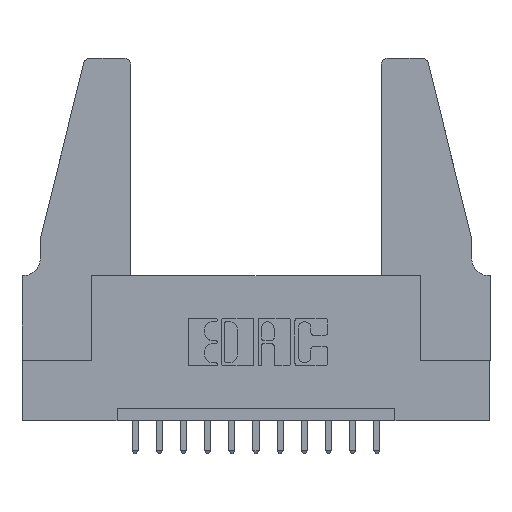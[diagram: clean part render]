
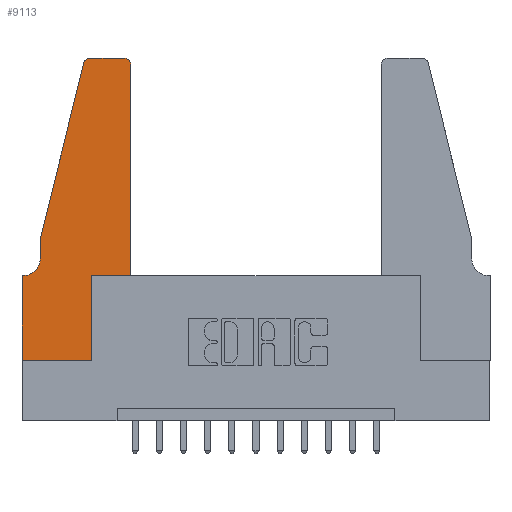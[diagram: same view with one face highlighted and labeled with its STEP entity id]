
A CAD part, top view. The second image highlights one B-rep face of the part: STEP entity #9113.
In plain terms, the highlighted planar face has unit normal (0, 0, 1).
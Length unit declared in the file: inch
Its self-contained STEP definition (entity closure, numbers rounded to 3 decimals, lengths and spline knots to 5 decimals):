
#125 = CARTESIAN_POINT ( 'NONE',  ( 0., 0., 0.37 ) ) ;
#191 = CARTESIAN_POINT ( 'NONE',  ( 0.2865, 0.35, 0.37 ) ) ;
#464 = EDGE_CURVE ( 'NONE', #8051, #4748, #11514, .T. ) ;
#526 = DIRECTION ( 'NONE',  ( 1., 0., 0. ) ) ;
#865 = CARTESIAN_POINT ( 'NONE',  ( 0.2605, 1.25, 0.37 ) ) ;
#1005 = CARTESIAN_POINT ( 'NONE',  ( 0.0755, 0.5, 0.37 ) ) ;
#1082 = AXIS2_PLACEMENT_3D ( 'NONE', #11860, #1566, #526 ) ;
#1183 = VERTEX_POINT ( 'NONE', #7033 ) ;
#1487 = LINE ( 'NONE', #8215, #7141 ) ;
#1566 = DIRECTION ( 'NONE',  ( 0., 0., 1. ) ) ;
#1735 = ORIENTED_EDGE ( 'NONE', *, *, #11050, .T. ) ;
#1861 = DIRECTION ( 'NONE',  ( -1., 0., 0. ) ) ;
#1981 = EDGE_CURVE ( 'NONE', #13325, #2441, #13966, .T. ) ;
#2212 = EDGE_CURVE ( 'NONE', #7018, #9167, #8469, .T. ) ;
#2230 = EDGE_CURVE ( 'NONE', #11353, #11783, #5502, .T. ) ;
#2374 = DIRECTION ( 'NONE',  ( 0., -1., 0. ) ) ;
#2427 = CARTESIAN_POINT ( 'NONE',  ( 0.2865, 0.35, 0.37 ) ) ;
#2441 = VERTEX_POINT ( 'NONE', #2914 ) ;
#2914 = CARTESIAN_POINT ( 'NONE',  ( 0.0755, 0.42, 0.37 ) ) ;
#3100 = DIRECTION ( 'NONE',  ( 0., 0., -1. ) ) ;
#3194 = VECTOR ( 'NONE', #1861, 39.37008 ) ;
#3404 = CIRCLE ( 'NONE', #1082, 0.03 ) ;
#3438 = CARTESIAN_POINT ( 'NONE',  ( 0.4505, 0.35, 0.37 ) ) ;
#3456 = EDGE_CURVE ( 'NONE', #7740, #13503, #10553, .T. ) ;
#3614 = LINE ( 'NONE', #125, #12261 ) ;
#3821 = DIRECTION ( 'NONE',  ( 0., 0., 1. ) ) ;
#4093 = EDGE_CURVE ( 'NONE', #2441, #1183, #4192, .T. ) ;
#4132 = DIRECTION ( 'NONE',  ( 1., 0., 0. ) ) ;
#4192 = CIRCLE ( 'NONE', #4378, 0.07 ) ;
#4266 = DIRECTION ( 'NONE',  ( -1., 0., 0. ) ) ;
#4378 = AXIS2_PLACEMENT_3D ( 'NONE', #9889, #3100, #4266 ) ;
#4401 = DIRECTION ( 'NONE',  ( 1., 0., 0. ) ) ;
#4481 = ORIENTED_EDGE ( 'NONE', *, *, #1981, .T. ) ;
#4527 = LINE ( 'NONE', #6327, #11199 ) ;
#4588 = DIRECTION ( 'NONE',  ( 0., 0., 1. ) ) ;
#4616 = FACE_OUTER_BOUND ( 'NONE', #8795, .T. ) ;
#4748 = VERTEX_POINT ( 'NONE', #6319 ) ;
#4884 = EDGE_CURVE ( 'NONE', #9167, #11353, #3614, .T. ) ;
#4938 = AXIS2_PLACEMENT_3D ( 'NONE', #10021, #4588, #4401 ) ;
#4947 = ORIENTED_EDGE ( 'NONE', *, *, #2212, .T. ) ;
#5011 = DIRECTION ( 'NONE',  ( 1., 0., 0. ) ) ;
#5020 = VECTOR ( 'NONE', #10306, 39.37008 ) ;
#5091 = VECTOR ( 'NONE', #9782, 39.37008 ) ;
#5502 = LINE ( 'NONE', #2427, #10417 ) ;
#5959 = CARTESIAN_POINT ( 'NONE',  ( 0.4205, 1.25, 0.37 ) ) ;
#6046 = DIRECTION ( 'NONE',  ( -1., 0., 0. ) ) ;
#6211 = ORIENTED_EDGE ( 'NONE', *, *, #3456, .T. ) ;
#6319 = CARTESIAN_POINT ( 'NONE',  ( 0.4505, 1.22, 0.37 ) ) ;
#6327 = CARTESIAN_POINT ( 'NONE',  ( 0.4505, 0.35, 0.37 ) ) ;
#6561 = EDGE_CURVE ( 'NONE', #4748, #8062, #3404, .T. ) ;
#7018 = VERTEX_POINT ( 'NONE', #11134 ) ;
#7033 = CARTESIAN_POINT ( 'NONE',  ( 0.0055, 0.35, 0.37 ) ) ;
#7141 = VECTOR ( 'NONE', #6046, 39.37008 ) ;
#7169 = EDGE_CURVE ( 'NONE', #8062, #7740, #10963, .T. ) ;
#7381 = ORIENTED_EDGE ( 'NONE', *, *, #4884, .T. ) ;
#7740 = VERTEX_POINT ( 'NONE', #9675 ) ;
#7977 = ORIENTED_EDGE ( 'NONE', *, *, #6561, .T. ) ;
#8051 = VERTEX_POINT ( 'NONE', #13981 ) ;
#8062 = VERTEX_POINT ( 'NONE', #5959 ) ;
#8207 = CARTESIAN_POINT ( 'NONE',  ( 0.25487, 1.22718, 0.37 ) ) ;
#8215 = CARTESIAN_POINT ( 'NONE',  ( 0.0755, 0.35, 0.37 ) ) ;
#8216 = ORIENTED_EDGE ( 'NONE', *, *, #464, .T. ) ;
#8361 = EDGE_CURVE ( 'NONE', #11783, #8051, #4527, .T. ) ;
#8469 = LINE ( 'NONE', #13426, #13411 ) ;
#8581 = LINE ( 'NONE', #14135, #5091 ) ;
#8644 = VECTOR ( 'NONE', #12544, 39.37008 ) ;
#8793 = AXIS2_PLACEMENT_3D ( 'NONE', #10623, #3821, #10670 ) ;
#8795 = EDGE_LOOP ( 'NONE', ( #14193, #6211, #1735, #4481, #13288, #11164, #4947, #7381, #9685, #11545, #8216, #7977 ) ) ;
#9113 = ADVANCED_FACE ( 'NONE', ( #4616 ), #10218, .T. ) ;
#9167 = VERTEX_POINT ( 'NONE', #11180 ) ;
#9238 = DIRECTION ( 'NONE',  ( 0., 1., 0. ) ) ;
#9675 = CARTESIAN_POINT ( 'NONE',  ( 0.284, 1.25, 0.37 ) ) ;
#9685 = ORIENTED_EDGE ( 'NONE', *, *, #2230, .T. ) ;
#9782 = DIRECTION ( 'NONE',  ( -0.239, -0.971, 0. ) ) ;
#9889 = CARTESIAN_POINT ( 'NONE',  ( 0.0055, 0.42, 0.37 ) ) ;
#10021 = CARTESIAN_POINT ( 'NONE',  ( 0., 0.35, 0.37 ) ) ;
#10218 = PLANE ( 'NONE',  #4938 ) ;
#10282 = CARTESIAN_POINT ( 'NONE',  ( 0.0755, 0.5, 0.37 ) ) ;
#10306 = DIRECTION ( 'NONE',  ( 0., 1., 0. ) ) ;
#10417 = VECTOR ( 'NONE', #9238, 39.37008 ) ;
#10553 = CIRCLE ( 'NONE', #8793, 0.03 ) ;
#10623 = CARTESIAN_POINT ( 'NONE',  ( 0.284, 1.22, 0.37 ) ) ;
#10670 = DIRECTION ( 'NONE',  ( 1., 0., 0. ) ) ;
#10963 = LINE ( 'NONE', #865, #3194 ) ;
#11050 = EDGE_CURVE ( 'NONE', #13503, #13325, #8581, .T. ) ;
#11134 = CARTESIAN_POINT ( 'NONE',  ( 0., 0.35, 0.37 ) ) ;
#11164 = ORIENTED_EDGE ( 'NONE', *, *, #13037, .T. ) ;
#11180 = CARTESIAN_POINT ( 'NONE',  ( 0., 0., 0.37 ) ) ;
#11199 = VECTOR ( 'NONE', #4132, 39.37008 ) ;
#11353 = VERTEX_POINT ( 'NONE', #13635 ) ;
#11514 = LINE ( 'NONE', #3438, #5020 ) ;
#11545 = ORIENTED_EDGE ( 'NONE', *, *, #8361, .T. ) ;
#11783 = VERTEX_POINT ( 'NONE', #191 ) ;
#11860 = CARTESIAN_POINT ( 'NONE',  ( 0.4205, 1.22, 0.37 ) ) ;
#12261 = VECTOR ( 'NONE', #5011, 39.37008 ) ;
#12544 = DIRECTION ( 'NONE',  ( 0., -1., 0. ) ) ;
#13037 = EDGE_CURVE ( 'NONE', #1183, #7018, #1487, .T. ) ;
#13288 = ORIENTED_EDGE ( 'NONE', *, *, #4093, .T. ) ;
#13325 = VERTEX_POINT ( 'NONE', #1005 ) ;
#13411 = VECTOR ( 'NONE', #2374, 39.37008 ) ;
#13426 = CARTESIAN_POINT ( 'NONE',  ( 0., 0., 0.37 ) ) ;
#13503 = VERTEX_POINT ( 'NONE', #8207 ) ;
#13635 = CARTESIAN_POINT ( 'NONE',  ( 0.2865, 0., 0.37 ) ) ;
#13966 = LINE ( 'NONE', #10282, #8644 ) ;
#13981 = CARTESIAN_POINT ( 'NONE',  ( 0.4505, 0.35, 0.37 ) ) ;
#14135 = CARTESIAN_POINT ( 'NONE',  ( 0.0755, 0.5, 0.37 ) ) ;
#14193 = ORIENTED_EDGE ( 'NONE', *, *, #7169, .T. ) ;
